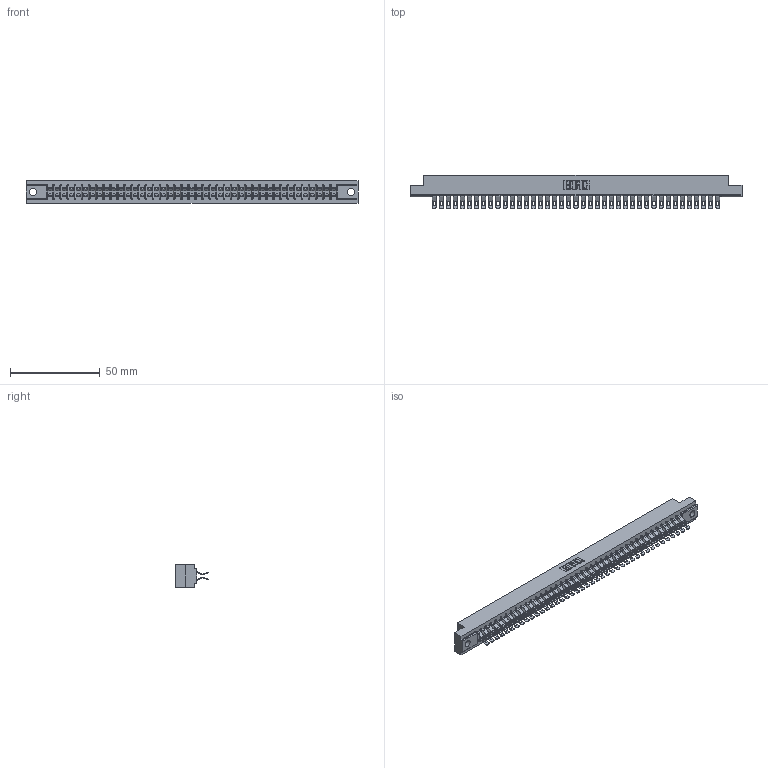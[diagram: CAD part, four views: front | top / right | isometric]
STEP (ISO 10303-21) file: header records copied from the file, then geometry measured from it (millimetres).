
FILE_DESCRIPTION (( 'STEP AP203' ), '1' );
FILE_NAME ('357-082-555-202.STEP', '2019-09-19T16:56:00', ( '' ), ( '' ), 'SwSTEP 2.0', 'SolidWorks 2016', '' );
FILE_SCHEMA (( 'CONFIG_CONTROL_DESIGN' ));
Length unit declared in the file: inch
Products named in the file (3): 307-290-001_555; 357-082-555-202; 307 Part_.128 Dia Mounting Holes
Assembly tree (83 placements, depth 2):
  357-082-555-202
    307 Part_.128 Dia Mounting Holes
    307-290-001_555  x82
Bounding box: 185.47 x 18.75 x 12.7 mm (x, y, z)
Volume: 19872 mm3; surface area: 25452 mm2
Topology: 83 solids, 83 shells, 5162 faces, 15165 edges, 9886 vertices
Faces by surface type: plane 2858, cylinder 2220, sphere 84
Entity records: 37123 total; most frequent: CARTESIAN_POINT 6077, ORIENTED_EDGE 6024, DIRECTION 5960, EDGE_CURVE 3012, LINE 2298, VECTOR 2298, VERTEX_POINT 1948, AXIS2_PLACEMENT_3D 1831
